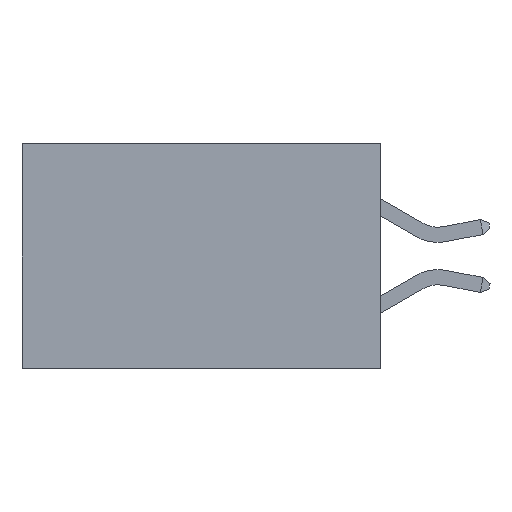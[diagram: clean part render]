
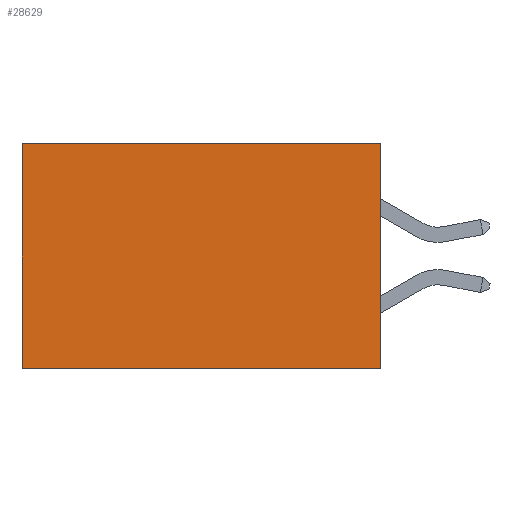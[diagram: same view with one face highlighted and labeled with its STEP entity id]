
A CAD part, left-side view. The second image highlights one B-rep face of the part: STEP entity #28629.
In plain terms, the highlighted planar face has unit normal (-1, 0, 0).
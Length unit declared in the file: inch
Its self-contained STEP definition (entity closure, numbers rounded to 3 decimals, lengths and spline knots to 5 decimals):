
#1641 = VERTEX_POINT ( 'NONE', #8264 ) ;
#3328 = CARTESIAN_POINT ( 'NONE',  ( 0.277, 0.59, -0.37 ) ) ;
#4467 = DIRECTION ( 'NONE',  ( 1., 0., 0. ) ) ;
#5025 = VERTEX_POINT ( 'NONE', #3328 ) ;
#5580 = EDGE_LOOP ( 'NONE', ( #29199, #26630, #21307, #16952 ) ) ;
#8264 = CARTESIAN_POINT ( 'NONE',  ( 0.277, 0., 0. ) ) ;
#9217 = CARTESIAN_POINT ( 'NONE',  ( 0.277, 0.59, 0. ) ) ;
#9441 = VECTOR ( 'NONE', #20596, 39.37008 ) ;
#12255 = PLANE ( 'NONE',  #24409 ) ;
#13167 = EDGE_CURVE ( 'NONE', #27811, #5025, #32761, .T. ) ;
#15062 = CARTESIAN_POINT ( 'NONE',  ( 0.277, 0.59, -0.37 ) ) ;
#15183 = LINE ( 'NONE', #27703, #22005 ) ;
#15560 = CARTESIAN_POINT ( 'NONE',  ( 0.277, 0., -0.37 ) ) ;
#16365 = LINE ( 'NONE', #33413, #9441 ) ;
#16952 = ORIENTED_EDGE ( 'NONE', *, *, #17823, .T. ) ;
#17807 = LINE ( 'NONE', #19871, #21047 ) ;
#17823 = EDGE_CURVE ( 'NONE', #1641, #27811, #15183, .T. ) ;
#17989 = EDGE_CURVE ( 'NONE', #28810, #5025, #16365, .T. ) ;
#19871 = CARTESIAN_POINT ( 'NONE',  ( 0.277, 0., -0.37 ) ) ;
#19927 = DIRECTION ( 'NONE',  ( 0., 1., 0. ) ) ;
#20044 = CARTESIAN_POINT ( 'NONE',  ( 0.277, 0., -0.37 ) ) ;
#20210 = DIRECTION ( 'NONE',  ( 0., 0., -1. ) ) ;
#20596 = DIRECTION ( 'NONE',  ( 0., 1., 0. ) ) ;
#21047 = VECTOR ( 'NONE', #25074, 39.37008 ) ;
#21307 = ORIENTED_EDGE ( 'NONE', *, *, #21363, .F. ) ;
#21363 = EDGE_CURVE ( 'NONE', #1641, #28810, #17807, .T. ) ;
#22005 = VECTOR ( 'NONE', #19927, 39.37008 ) ;
#22637 = DIRECTION ( 'NONE',  ( 0., 0., -1. ) ) ;
#24409 = AXIS2_PLACEMENT_3D ( 'NONE', #20044, #4467, #22637 ) ;
#25074 = DIRECTION ( 'NONE',  ( 0., 0., -1. ) ) ;
#25142 = VECTOR ( 'NONE', #20210, 39.37008 ) ;
#26053 = FACE_OUTER_BOUND ( 'NONE', #5580, .T. ) ;
#26630 = ORIENTED_EDGE ( 'NONE', *, *, #17989, .F. ) ;
#27703 = CARTESIAN_POINT ( 'NONE',  ( 0.277, 0., 0. ) ) ;
#27811 = VERTEX_POINT ( 'NONE', #9217 ) ;
#28629 = ADVANCED_FACE ( 'NONE', ( #26053 ), #12255, .F. ) ;
#28810 = VERTEX_POINT ( 'NONE', #15560 ) ;
#29199 = ORIENTED_EDGE ( 'NONE', *, *, #13167, .T. ) ;
#32761 = LINE ( 'NONE', #15062, #25142 ) ;
#33413 = CARTESIAN_POINT ( 'NONE',  ( 0.277, 0., -0.37 ) ) ;
